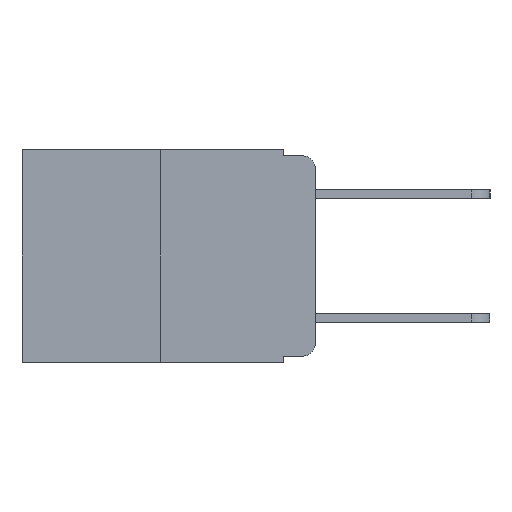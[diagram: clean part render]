
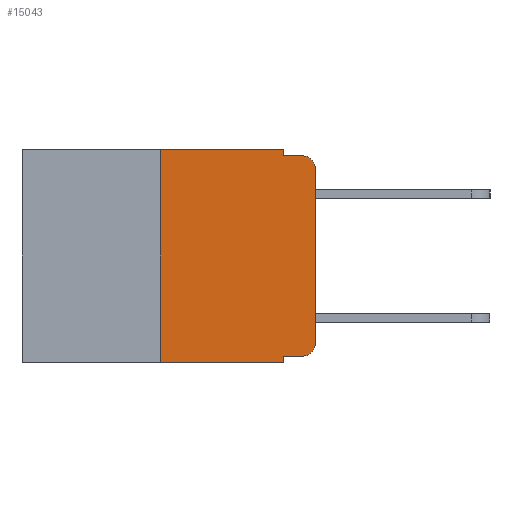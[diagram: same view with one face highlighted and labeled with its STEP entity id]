
A CAD part, left-side view. The second image highlights one B-rep face of the part: STEP entity #15043.
In plain terms, the highlighted planar face has unit normal (-1, 0, 0).
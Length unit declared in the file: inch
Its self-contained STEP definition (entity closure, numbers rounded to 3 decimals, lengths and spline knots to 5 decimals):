
#50 = EDGE_CURVE ( 'NONE', #12495, #12198, #22875, .T. ) ;
#261 = VERTEX_POINT ( 'NONE', #14517 ) ;
#905 = VECTOR ( 'NONE', #3837, 39.37008 ) ;
#1326 = EDGE_CURVE ( 'NONE', #12593, #16884, #1369, .T. ) ;
#1369 = LINE ( 'NONE', #2429, #10461 ) ;
#1695 = CARTESIAN_POINT ( 'NONE',  ( 0., 0.02, -0.333 ) ) ;
#1845 = VERTEX_POINT ( 'NONE', #4255 ) ;
#2152 = CARTESIAN_POINT ( 'NONE',  ( 0., 0., -0.03 ) ) ;
#2429 = CARTESIAN_POINT ( 'NONE',  ( 0., 0.051, 0. ) ) ;
#2463 = ORIENTED_EDGE ( 'NONE', *, *, #1326, .F. ) ;
#2489 = CARTESIAN_POINT ( 'NONE',  ( 0., 0.25, 0. ) ) ;
#2776 = DIRECTION ( 'NONE',  ( -1., 0., 0. ) ) ;
#2851 = DIRECTION ( 'NONE',  ( 0., 0., -1. ) ) ;
#2998 = VERTEX_POINT ( 'NONE', #6465 ) ;
#3160 = ORIENTED_EDGE ( 'NONE', *, *, #16206, .T. ) ;
#3237 = EDGE_CURVE ( 'NONE', #16884, #261, #10566, .T. ) ;
#3240 = CARTESIAN_POINT ( 'NONE',  ( 0., 0.25, 0. ) ) ;
#3563 = LINE ( 'NONE', #2489, #21872 ) ;
#3699 = PLANE ( 'NONE',  #10815 ) ;
#3774 = DIRECTION ( 'NONE',  ( 0., -1., 0. ) ) ;
#3837 = DIRECTION ( 'NONE',  ( 0., -1., 0. ) ) ;
#4161 = VECTOR ( 'NONE', #17286, 39.37008 ) ;
#4223 = CARTESIAN_POINT ( 'NONE',  ( 0., 0.051, 0. ) ) ;
#4255 = CARTESIAN_POINT ( 'NONE',  ( 0., 0.051, -0.333 ) ) ;
#5437 = CARTESIAN_POINT ( 'NONE',  ( 0., 0.473, -0.343 ) ) ;
#5532 = DIRECTION ( 'NONE',  ( 0., 0., -1. ) ) ;
#5796 = CARTESIAN_POINT ( 'NONE',  ( 0., 0.25, -0.343 ) ) ;
#6160 = DIRECTION ( 'NONE',  ( 0., 0., 1. ) ) ;
#6465 = CARTESIAN_POINT ( 'NONE',  ( 0., 0., -0.313 ) ) ;
#6971 = ORIENTED_EDGE ( 'NONE', *, *, #14353, .T. ) ;
#7751 = EDGE_LOOP ( 'NONE', ( #3160, #17779, #16715, #2463, #16978, #12888, #8717, #15361, #21026, #6971 ) ) ;
#7918 = EDGE_CURVE ( 'NONE', #21523, #261, #10349, .T. ) ;
#8686 = VECTOR ( 'NONE', #22505, 39.37008 ) ;
#8717 = ORIENTED_EDGE ( 'NONE', *, *, #50, .T. ) ;
#8831 = VECTOR ( 'NONE', #3774, 39.37008 ) ;
#9010 = CARTESIAN_POINT ( 'NONE',  ( 0., 0.02, -0.313 ) ) ;
#10088 = LINE ( 'NONE', #19807, #14226 ) ;
#10349 = CIRCLE ( 'NONE', #15838, 0.02 ) ;
#10461 = VECTOR ( 'NONE', #2851, 39.37008 ) ;
#10566 = LINE ( 'NONE', #14545, #905 ) ;
#10815 = AXIS2_PLACEMENT_3D ( 'NONE', #18964, #16186, #5532 ) ;
#10816 = DIRECTION ( 'NONE',  ( 0., 0., -1. ) ) ;
#10820 = CARTESIAN_POINT ( 'NONE',  ( 0., 0., 0. ) ) ;
#12016 = CARTESIAN_POINT ( 'NONE',  ( 0., 0.051, -0.333 ) ) ;
#12198 = VERTEX_POINT ( 'NONE', #15626 ) ;
#12495 = VERTEX_POINT ( 'NONE', #5796 ) ;
#12593 = VERTEX_POINT ( 'NONE', #4223 ) ;
#12605 = DIRECTION ( 'NONE',  ( 0., 0., 1. ) ) ;
#12754 = DIRECTION ( 'NONE',  ( 0., -1., 0. ) ) ;
#12888 = ORIENTED_EDGE ( 'NONE', *, *, #15244, .F. ) ;
#13418 = CARTESIAN_POINT ( 'NONE',  ( 0., 0.051, -0.01 ) ) ;
#13548 = CARTESIAN_POINT ( 'NONE',  ( 0., 0.02, -0.03 ) ) ;
#14226 = VECTOR ( 'NONE', #12754, 39.37008 ) ;
#14353 = EDGE_CURVE ( 'NONE', #20758, #2998, #21918, .T. ) ;
#14440 = VECTOR ( 'NONE', #12605, 39.37008 ) ;
#14517 = CARTESIAN_POINT ( 'NONE',  ( 0., 0.02, -0.01 ) ) ;
#14545 = CARTESIAN_POINT ( 'NONE',  ( 0., 0.051, -0.01 ) ) ;
#14801 = EDGE_CURVE ( 'NONE', #1845, #12198, #18345, .T. ) ;
#15043 = ADVANCED_FACE ( 'NONE', ( #18054 ), #3699, .F. ) ;
#15244 = EDGE_CURVE ( 'NONE', #12495, #17775, #3563, .T. ) ;
#15321 = DIRECTION ( 'NONE',  ( 0., 0., -1. ) ) ;
#15361 = ORIENTED_EDGE ( 'NONE', *, *, #14801, .F. ) ;
#15517 = CARTESIAN_POINT ( 'NONE',  ( 0., 0.051, 0. ) ) ;
#15626 = CARTESIAN_POINT ( 'NONE',  ( 0., 0.051, -0.343 ) ) ;
#15838 = AXIS2_PLACEMENT_3D ( 'NONE', #13548, #2776, #15321 ) ;
#16083 = LINE ( 'NONE', #10820, #14440 ) ;
#16186 = DIRECTION ( 'NONE',  ( 1., 0., 0. ) ) ;
#16206 = EDGE_CURVE ( 'NONE', #2998, #21523, #16083, .T. ) ;
#16715 = ORIENTED_EDGE ( 'NONE', *, *, #3237, .F. ) ;
#16884 = VERTEX_POINT ( 'NONE', #13418 ) ;
#16978 = ORIENTED_EDGE ( 'NONE', *, *, #20843, .F. ) ;
#17286 = DIRECTION ( 'NONE',  ( 0., 0., -1. ) ) ;
#17775 = VERTEX_POINT ( 'NONE', #3240 ) ;
#17779 = ORIENTED_EDGE ( 'NONE', *, *, #7918, .T. ) ;
#18054 = FACE_OUTER_BOUND ( 'NONE', #7751, .T. ) ;
#18073 = LINE ( 'NONE', #12016, #8686 ) ;
#18345 = LINE ( 'NONE', #15517, #4161 ) ;
#18964 = CARTESIAN_POINT ( 'NONE',  ( 0., 0.473, 0. ) ) ;
#19807 = CARTESIAN_POINT ( 'NONE',  ( 0., 0.473, 0. ) ) ;
#20384 = AXIS2_PLACEMENT_3D ( 'NONE', #9010, #21322, #10816 ) ;
#20665 = EDGE_CURVE ( 'NONE', #1845, #20758, #18073, .T. ) ;
#20758 = VERTEX_POINT ( 'NONE', #1695 ) ;
#20843 = EDGE_CURVE ( 'NONE', #17775, #12593, #10088, .T. ) ;
#21026 = ORIENTED_EDGE ( 'NONE', *, *, #20665, .T. ) ;
#21322 = DIRECTION ( 'NONE',  ( -1., 0., 0. ) ) ;
#21523 = VERTEX_POINT ( 'NONE', #2152 ) ;
#21872 = VECTOR ( 'NONE', #6160, 39.37008 ) ;
#21918 = CIRCLE ( 'NONE', #20384, 0.02 ) ;
#22505 = DIRECTION ( 'NONE',  ( 0., -1., 0. ) ) ;
#22875 = LINE ( 'NONE', #5437, #8831 ) ;
